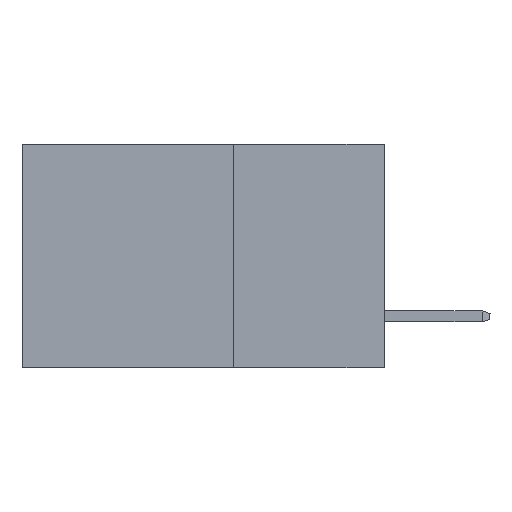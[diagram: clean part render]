
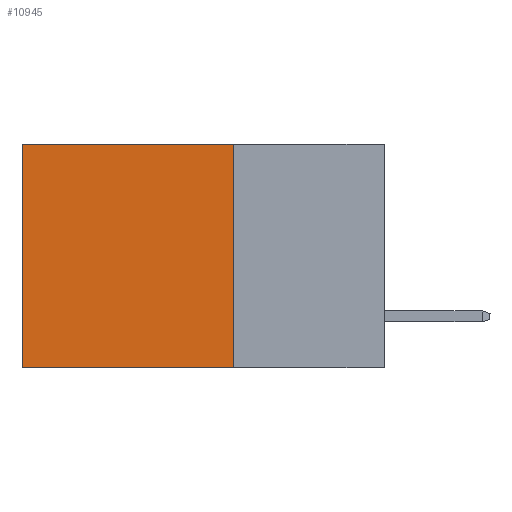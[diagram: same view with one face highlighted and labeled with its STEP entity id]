
A CAD part, left-side view. The second image highlights one B-rep face of the part: STEP entity #10945.
In plain terms, the highlighted planar face has unit normal (-1, 0, 0).
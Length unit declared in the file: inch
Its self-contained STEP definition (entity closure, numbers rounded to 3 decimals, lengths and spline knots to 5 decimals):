
#233 = ORIENTED_EDGE ( 'NONE', *, *, #7796, .F. ) ;
#444 = EDGE_CURVE ( 'NONE', #12952, #4200, #14043, .T. ) ;
#1042 = VERTEX_POINT ( 'NONE', #12290 ) ;
#1932 = DIRECTION ( 'NONE',  ( 0., 1., 0. ) ) ;
#3450 = ORIENTED_EDGE ( 'NONE', *, *, #12736, .T. ) ;
#3649 = EDGE_CURVE ( 'NONE', #7473, #4200, #10812, .T. ) ;
#4200 = VERTEX_POINT ( 'NONE', #14371 ) ;
#4357 = DIRECTION ( 'NONE',  ( 0., 1., 0. ) ) ;
#4569 = PLANE ( 'NONE',  #7817 ) ;
#4955 = DIRECTION ( 'NONE',  ( 0., 0., -1. ) ) ;
#5354 = DIRECTION ( 'NONE',  ( 0., 0., -1. ) ) ;
#5365 = VECTOR ( 'NONE', #4955, 39.37008 ) ;
#5507 = CARTESIAN_POINT ( 'NONE',  ( 0.2615, 0.25, -0.37 ) ) ;
#7473 = VERTEX_POINT ( 'NONE', #8088 ) ;
#7520 = CARTESIAN_POINT ( 'NONE',  ( 0.2615, 0.25, -0.37 ) ) ;
#7796 = EDGE_CURVE ( 'NONE', #1042, #12952, #9871, .T. ) ;
#7817 = AXIS2_PLACEMENT_3D ( 'NONE', #7520, #11992, #13865 ) ;
#8088 = CARTESIAN_POINT ( 'NONE',  ( 0.2615, 0.6, 0. ) ) ;
#8523 = CARTESIAN_POINT ( 'NONE',  ( 0.2615, 0.6, -0.37 ) ) ;
#9655 = ORIENTED_EDGE ( 'NONE', *, *, #444, .F. ) ;
#9871 = LINE ( 'NONE', #5507, #10162 ) ;
#10125 = CARTESIAN_POINT ( 'NONE',  ( 0.2615, 0.25, -0.37 ) ) ;
#10162 = VECTOR ( 'NONE', #5354, 39.37008 ) ;
#10357 = FACE_OUTER_BOUND ( 'NONE', #10942, .T. ) ;
#10812 = LINE ( 'NONE', #8523, #5365 ) ;
#10942 = EDGE_LOOP ( 'NONE', ( #13554, #9655, #233, #3450 ) ) ;
#10945 = ADVANCED_FACE ( 'NONE', ( #10357 ), #4569, .F. ) ;
#11453 = VECTOR ( 'NONE', #4357, 39.37008 ) ;
#11992 = DIRECTION ( 'NONE',  ( 1., 0., 0. ) ) ;
#12173 = CARTESIAN_POINT ( 'NONE',  ( 0.2615, 0.25, -0.37 ) ) ;
#12290 = CARTESIAN_POINT ( 'NONE',  ( 0.2615, 0.25, 0. ) ) ;
#12736 = EDGE_CURVE ( 'NONE', #1042, #7473, #12744, .T. ) ;
#12742 = VECTOR ( 'NONE', #1932, 39.37008 ) ;
#12744 = LINE ( 'NONE', #13920, #12742 ) ;
#12952 = VERTEX_POINT ( 'NONE', #10125 ) ;
#13554 = ORIENTED_EDGE ( 'NONE', *, *, #3649, .T. ) ;
#13865 = DIRECTION ( 'NONE',  ( 0., 0., -1. ) ) ;
#13920 = CARTESIAN_POINT ( 'NONE',  ( 0.2615, 0.25, 0. ) ) ;
#14043 = LINE ( 'NONE', #12173, #11453 ) ;
#14371 = CARTESIAN_POINT ( 'NONE',  ( 0.2615, 0.6, -0.37 ) ) ;
